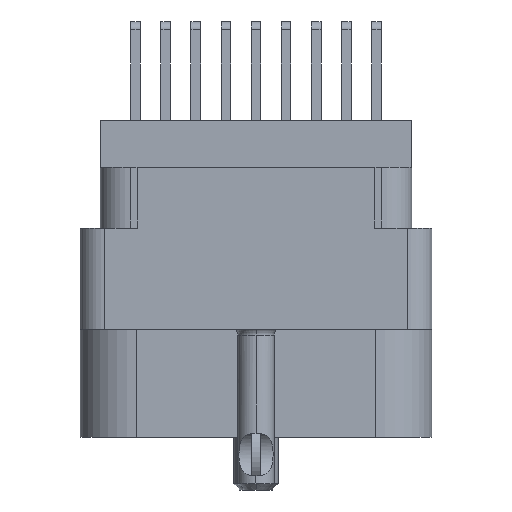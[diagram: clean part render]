
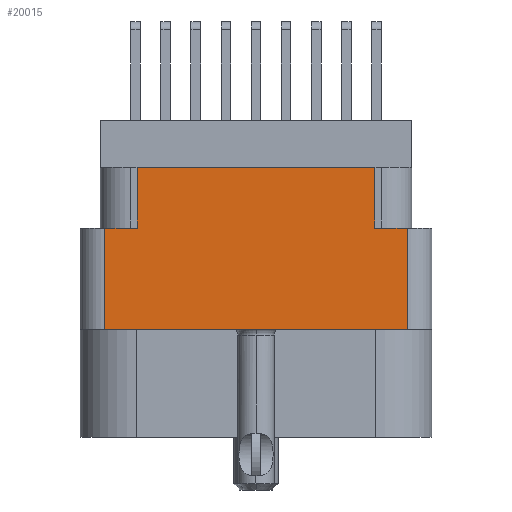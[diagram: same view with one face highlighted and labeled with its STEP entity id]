
A CAD part, left-side view. The second image highlights one B-rep face of the part: STEP entity #20015.
In plain terms, the highlighted planar face has unit normal (-1, 0, 0).
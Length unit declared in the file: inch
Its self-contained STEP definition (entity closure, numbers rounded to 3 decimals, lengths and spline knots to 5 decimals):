
#493 = VERTEX_POINT ( 'NONE', #38745 ) ;
#720 = DIRECTION ( 'NONE',  ( 0., 0., 1. ) ) ;
#1226 = DIRECTION ( 'NONE',  ( 0., -1., 0. ) ) ;
#1263 = VERTEX_POINT ( 'NONE', #22427 ) ;
#1484 = VECTOR ( 'NONE', #11720, 39.37008 ) ;
#1541 = VECTOR ( 'NONE', #33590, 39.37008 ) ;
#1558 = AXIS2_PLACEMENT_3D ( 'NONE', #36589, #33029, #720 ) ;
#2448 = CARTESIAN_POINT ( 'NONE',  ( -1., 0.376, -0.52 ) ) ;
#2609 = EDGE_CURVE ( 'NONE', #37484, #26534, #44257, .T. ) ;
#6482 = CARTESIAN_POINT ( 'NONE',  ( -1., 0., -0.52 ) ) ;
#6860 = DIRECTION ( 'NONE',  ( 0., -1., 0. ) ) ;
#7300 = CARTESIAN_POINT ( 'NONE',  ( -1., -0.376, -0.789 ) ) ;
#7711 = CARTESIAN_POINT ( 'NONE',  ( -1., 0.296, -0.117 ) ) ;
#7955 = EDGE_CURVE ( 'NONE', #26534, #15058, #39021, .T. ) ;
#8456 = VECTOR ( 'NONE', #26803, 39.37008 ) ;
#8476 = ORIENTED_EDGE ( 'NONE', *, *, #14999, .F. ) ;
#9592 = CARTESIAN_POINT ( 'NONE',  ( -1., 0.376, -0.268 ) ) ;
#10173 = VERTEX_POINT ( 'NONE', #7711 ) ;
#10832 = VECTOR ( 'NONE', #6860, 39.37008 ) ;
#11720 = DIRECTION ( 'NONE',  ( 0., 0., -1. ) ) ;
#13575 = ORIENTED_EDGE ( 'NONE', *, *, #21489, .F. ) ;
#14622 = CARTESIAN_POINT ( 'NONE',  ( -1., 0., -0.268 ) ) ;
#14678 = CARTESIAN_POINT ( 'NONE',  ( -1., 0.438, -0.117 ) ) ;
#14999 = EDGE_CURVE ( 'NONE', #10173, #493, #25624, .T. ) ;
#15058 = VERTEX_POINT ( 'NONE', #38837 ) ;
#17396 = DIRECTION ( 'NONE',  ( 0., -1., 0. ) ) ;
#18235 = LINE ( 'NONE', #7300, #29857 ) ;
#20015 = ADVANCED_FACE ( 'NONE', ( #29449 ), #37055, .T. ) ;
#20225 = VERTEX_POINT ( 'NONE', #30751 ) ;
#20303 = DIRECTION ( 'NONE',  ( 0., 0., 1. ) ) ;
#20477 = VECTOR ( 'NONE', #1226, 39.37008 ) ;
#21489 = EDGE_CURVE ( 'NONE', #1263, #10173, #23924, .T. ) ;
#21801 = DIRECTION ( 'NONE',  ( 0., 0., 1. ) ) ;
#22207 = CARTESIAN_POINT ( 'NONE',  ( -1., 0.376, -0.789 ) ) ;
#22427 = CARTESIAN_POINT ( 'NONE',  ( -1., 0.296, -0.268 ) ) ;
#22869 = EDGE_CURVE ( 'NONE', #29381, #493, #23398, .T. ) ;
#23398 = LINE ( 'NONE', #31241, #44561 ) ;
#23924 = LINE ( 'NONE', #45754, #8456 ) ;
#25624 = LINE ( 'NONE', #14678, #10832 ) ;
#25822 = EDGE_CURVE ( 'NONE', #29381, #20225, #29140, .T. ) ;
#25939 = EDGE_CURVE ( 'NONE', #37484, #1263, #33759, .T. ) ;
#26348 = ORIENTED_EDGE ( 'NONE', *, *, #31121, .T. ) ;
#26534 = VERTEX_POINT ( 'NONE', #2448 ) ;
#26803 = DIRECTION ( 'NONE',  ( 0., 0., 1. ) ) ;
#29140 = LINE ( 'NONE', #14622, #1541 ) ;
#29166 = ORIENTED_EDGE ( 'NONE', *, *, #7955, .T. ) ;
#29381 = VERTEX_POINT ( 'NONE', #35431 ) ;
#29449 = FACE_OUTER_BOUND ( 'NONE', #31511, .T. ) ;
#29857 = VECTOR ( 'NONE', #21801, 39.37008 ) ;
#29930 = ORIENTED_EDGE ( 'NONE', *, *, #22869, .T. ) ;
#30751 = CARTESIAN_POINT ( 'NONE',  ( -1., -0.376, -0.268 ) ) ;
#31121 = EDGE_CURVE ( 'NONE', #15058, #20225, #18235, .T. ) ;
#31241 = CARTESIAN_POINT ( 'NONE',  ( -1., -0.296, -0.268 ) ) ;
#31511 = EDGE_LOOP ( 'NONE', ( #35831, #46726, #29166, #26348, #39896, #29930, #8476, #13575 ) ) ;
#33029 = DIRECTION ( 'NONE',  ( -1., 0., 0. ) ) ;
#33590 = DIRECTION ( 'NONE',  ( 0., -1., 0. ) ) ;
#33759 = LINE ( 'NONE', #41108, #20477 ) ;
#35431 = CARTESIAN_POINT ( 'NONE',  ( -1., -0.296, -0.268 ) ) ;
#35831 = ORIENTED_EDGE ( 'NONE', *, *, #25939, .F. ) ;
#36133 = VECTOR ( 'NONE', #17396, 39.37008 ) ;
#36589 = CARTESIAN_POINT ( 'NONE',  ( -1., -0.438, -0.789 ) ) ;
#37055 = PLANE ( 'NONE',  #1558 ) ;
#37484 = VERTEX_POINT ( 'NONE', #9592 ) ;
#38745 = CARTESIAN_POINT ( 'NONE',  ( -1., -0.296, -0.117 ) ) ;
#38837 = CARTESIAN_POINT ( 'NONE',  ( -1., -0.376, -0.52 ) ) ;
#39021 = LINE ( 'NONE', #6482, #36133 ) ;
#39896 = ORIENTED_EDGE ( 'NONE', *, *, #25822, .F. ) ;
#41108 = CARTESIAN_POINT ( 'NONE',  ( -1., 0., -0.268 ) ) ;
#44257 = LINE ( 'NONE', #22207, #1484 ) ;
#44561 = VECTOR ( 'NONE', #20303, 39.37008 ) ;
#45754 = CARTESIAN_POINT ( 'NONE',  ( -1., 0.296, -0.268 ) ) ;
#46726 = ORIENTED_EDGE ( 'NONE', *, *, #2609, .T. ) ;
